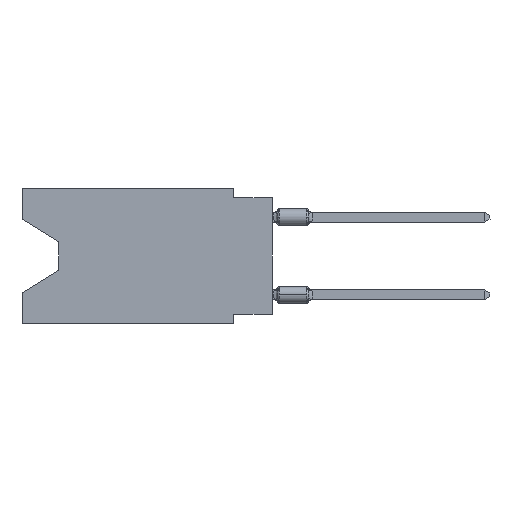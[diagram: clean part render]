
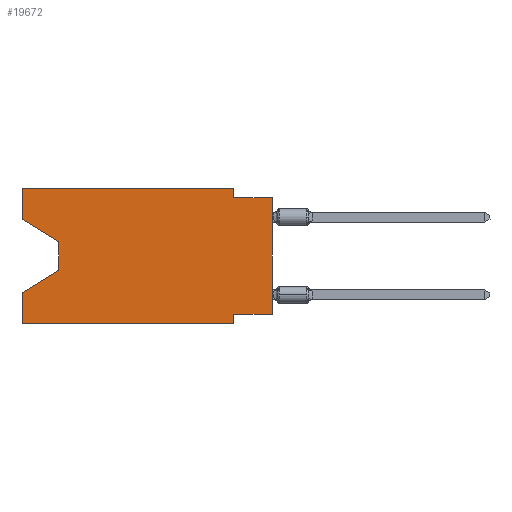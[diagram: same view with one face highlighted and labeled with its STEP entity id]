
A CAD part, left-side view. The second image highlights one B-rep face of the part: STEP entity #19672.
In plain terms, the highlighted planar face has unit normal (-1, 0, 0).
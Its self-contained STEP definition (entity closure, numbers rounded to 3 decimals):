
#310 = DIRECTION ( 'NONE',  ( 1., 0., 0. ) ) ;
#331 = CARTESIAN_POINT ( 'NONE',  ( 0., 16.383, -2.038 ) ) ;
#658 = CARTESIAN_POINT ( 'NONE',  ( 0., 0., -8.255 ) ) ;
#710 = CARTESIAN_POINT ( 'NONE',  ( 0., 16.383, 0. ) ) ;
#798 = VECTOR ( 'NONE', #11186, 1000. ) ;
#946 = CARTESIAN_POINT ( 'NONE',  ( 0., 13.97, -5.385 ) ) ;
#1007 = ORIENTED_EDGE ( 'NONE', *, *, #15093, .F. ) ;
#1023 = LINE ( 'NONE', #4928, #7936 ) ;
#1821 = VECTOR ( 'NONE', #6921, 1000. ) ;
#2269 = DIRECTION ( 'NONE',  ( 0., 0., -1. ) ) ;
#2516 = CARTESIAN_POINT ( 'NONE',  ( 0., 16.383, -8.89 ) ) ;
#2863 = EDGE_CURVE ( 'NONE', #16293, #6824, #26261, .T. ) ;
#3005 = VECTOR ( 'NONE', #21098, 1000. ) ;
#3291 = LINE ( 'NONE', #11598, #5261 ) ;
#3522 = LINE ( 'NONE', #22662, #23360 ) ;
#3539 = ORIENTED_EDGE ( 'NONE', *, *, #25217, .T. ) ;
#3657 = CARTESIAN_POINT ( 'NONE',  ( 0., 2.54, -8.255 ) ) ;
#4304 = CARTESIAN_POINT ( 'NONE',  ( 0., 0., 0. ) ) ;
#4498 = CARTESIAN_POINT ( 'NONE',  ( 0., 2.54, -8.89 ) ) ;
#4643 = DIRECTION ( 'NONE',  ( 0., -1., 0. ) ) ;
#4928 = CARTESIAN_POINT ( 'NONE',  ( 0., 13.97, -3.505 ) ) ;
#5105 = VERTEX_POINT ( 'NONE', #26725 ) ;
#5261 = VECTOR ( 'NONE', #5642, 1000. ) ;
#5519 = CARTESIAN_POINT ( 'NONE',  ( 0., 2.54, 0. ) ) ;
#5642 = DIRECTION ( 'NONE',  ( 0., -1., 0. ) ) ;
#6679 = EDGE_CURVE ( 'NONE', #12381, #26372, #23642, .T. ) ;
#6824 = VERTEX_POINT ( 'NONE', #14219 ) ;
#6921 = DIRECTION ( 'NONE',  ( 0., 0., 1. ) ) ;
#6939 = DIRECTION ( 'NONE',  ( 0., 0.855, -0.519 ) ) ;
#6961 = FACE_OUTER_BOUND ( 'NONE', #8471, .T. ) ;
#7337 = VECTOR ( 'NONE', #13839, 1000. ) ;
#7438 = EDGE_CURVE ( 'NONE', #20257, #23119, #19282, .T. ) ;
#7917 = VECTOR ( 'NONE', #4643, 1000. ) ;
#7937 = ORIENTED_EDGE ( 'NONE', *, *, #26240, .F. ) ;
#7936 = VECTOR ( 'NONE', #11699, 1000. ) ;
#8122 = VERTEX_POINT ( 'NONE', #4498 ) ;
#8471 = EDGE_LOOP ( 'NONE', ( #8497, #3539, #9481, #7937, #24584, #26442, #1007, #9395, #14752, #26253, #18254, #21875 ) ) ;
#8497 = ORIENTED_EDGE ( 'NONE', *, *, #2863, .T. ) ;
#8566 = CARTESIAN_POINT ( 'NONE',  ( 0., 0., -0.635 ) ) ;
#8714 = VERTEX_POINT ( 'NONE', #2516 ) ;
#9002 = EDGE_CURVE ( 'NONE', #5105, #26372, #19545, .T. ) ;
#9395 = ORIENTED_EDGE ( 'NONE', *, *, #9002, .T. ) ;
#9481 = ORIENTED_EDGE ( 'NONE', *, *, #7438, .T. ) ;
#9895 = DIRECTION ( 'NONE',  ( 0., 0., -1. ) ) ;
#10769 = EDGE_CURVE ( 'NONE', #8714, #8122, #10914, .T. ) ;
#10914 = LINE ( 'NONE', #19375, #798 ) ;
#11167 = CARTESIAN_POINT ( 'NONE',  ( 0., 2.54, -0.635 ) ) ;
#11186 = DIRECTION ( 'NONE',  ( 0., -1., 0. ) ) ;
#11287 = CARTESIAN_POINT ( 'NONE',  ( 0., 0., -0.635 ) ) ;
#11598 = CARTESIAN_POINT ( 'NONE',  ( 0., 16.383, 0. ) ) ;
#11699 = DIRECTION ( 'NONE',  ( 0., 0., -1. ) ) ;
#11989 = EDGE_CURVE ( 'NONE', #27172, #20116, #3291, .T. ) ;
#12183 = VECTOR ( 'NONE', #19729, 1000. ) ;
#12381 = VERTEX_POINT ( 'NONE', #11167 ) ;
#12645 = CARTESIAN_POINT ( 'NONE',  ( 0., 2.54, -8.89 ) ) ;
#13839 = DIRECTION ( 'NONE',  ( 0., 1., 0. ) ) ;
#14219 = CARTESIAN_POINT ( 'NONE',  ( 0., 13.97, -3.505 ) ) ;
#14277 = LINE ( 'NONE', #26492, #19937 ) ;
#14752 = ORIENTED_EDGE ( 'NONE', *, *, #6679, .F. ) ;
#15093 = EDGE_CURVE ( 'NONE', #5105, #18264, #26608, .T. ) ;
#15814 = CARTESIAN_POINT ( 'NONE',  ( 0., 16.383, 0. ) ) ;
#16293 = VERTEX_POINT ( 'NONE', #24398 ) ;
#16880 = EDGE_CURVE ( 'NONE', #20116, #12381, #3522, .T. ) ;
#18254 = ORIENTED_EDGE ( 'NONE', *, *, #11989, .F. ) ;
#18264 = VERTEX_POINT ( 'NONE', #3657 ) ;
#19282 = LINE ( 'NONE', #25684, #20791 ) ;
#19301 = PLANE ( 'NONE',  #24950 ) ;
#19375 = CARTESIAN_POINT ( 'NONE',  ( 0., 16.383, -8.89 ) ) ;
#19545 = LINE ( 'NONE', #4304, #1821 ) ;
#19672 = ADVANCED_FACE ( 'NONE', ( #6961 ), #19301, .F. ) ;
#19689 = DIRECTION ( 'NONE',  ( 0., 0., 1. ) ) ;
#19729 = DIRECTION ( 'NONE',  ( 0., -0.855, -0.519 ) ) ;
#19937 = VECTOR ( 'NONE', #22313, 1000. ) ;
#20116 = VERTEX_POINT ( 'NONE', #5519 ) ;
#20257 = VERTEX_POINT ( 'NONE', #946 ) ;
#20700 = LINE ( 'NONE', #12645, #3005 ) ;
#20791 = VECTOR ( 'NONE', #6939, 1000. ) ;
#21098 = DIRECTION ( 'NONE',  ( 0., 0., -1. ) ) ;
#21167 = VECTOR ( 'NONE', #19689, 1000. ) ;
#21364 = CARTESIAN_POINT ( 'NONE',  ( 0., 16.383, 0. ) ) ;
#21875 = ORIENTED_EDGE ( 'NONE', *, *, #27176, .F. ) ;
#22188 = LINE ( 'NONE', #15814, #21167 ) ;
#22313 = DIRECTION ( 'NONE',  ( 0., 0., 1. ) ) ;
#22662 = CARTESIAN_POINT ( 'NONE',  ( 0., 2.54, 0. ) ) ;
#23119 = VERTEX_POINT ( 'NONE', #25174 ) ;
#23360 = VECTOR ( 'NONE', #9895, 1000. ) ;
#23605 = EDGE_CURVE ( 'NONE', #18264, #8122, #20700, .T. ) ;
#23642 = LINE ( 'NONE', #11287, #7917 ) ;
#24398 = CARTESIAN_POINT ( 'NONE',  ( 0., 16.383, -2.038 ) ) ;
#24584 = ORIENTED_EDGE ( 'NONE', *, *, #10769, .T. ) ;
#24950 = AXIS2_PLACEMENT_3D ( 'NONE', #710, #310, #2269 ) ;
#25174 = CARTESIAN_POINT ( 'NONE',  ( 0., 16.383, -6.852 ) ) ;
#25217 = EDGE_CURVE ( 'NONE', #6824, #20257, #1023, .T. ) ;
#25684 = CARTESIAN_POINT ( 'NONE',  ( 0., 13.97, -5.385 ) ) ;
#26240 = EDGE_CURVE ( 'NONE', #8714, #23119, #14277, .T. ) ;
#26253 = ORIENTED_EDGE ( 'NONE', *, *, #16880, .F. ) ;
#26261 = LINE ( 'NONE', #331, #12183 ) ;
#26372 = VERTEX_POINT ( 'NONE', #8566 ) ;
#26442 = ORIENTED_EDGE ( 'NONE', *, *, #23605, .F. ) ;
#26492 = CARTESIAN_POINT ( 'NONE',  ( 0., 16.383, 0. ) ) ;
#26608 = LINE ( 'NONE', #658, #7337 ) ;
#26725 = CARTESIAN_POINT ( 'NONE',  ( 0., 0., -8.255 ) ) ;
#27172 = VERTEX_POINT ( 'NONE', #21364 ) ;
#27176 = EDGE_CURVE ( 'NONE', #16293, #27172, #22188, .T. ) ;
